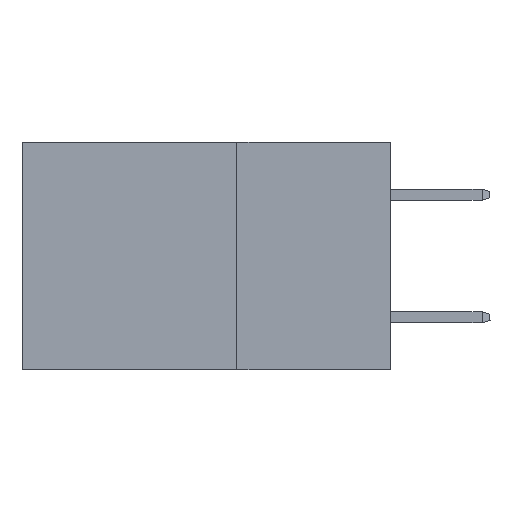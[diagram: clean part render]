
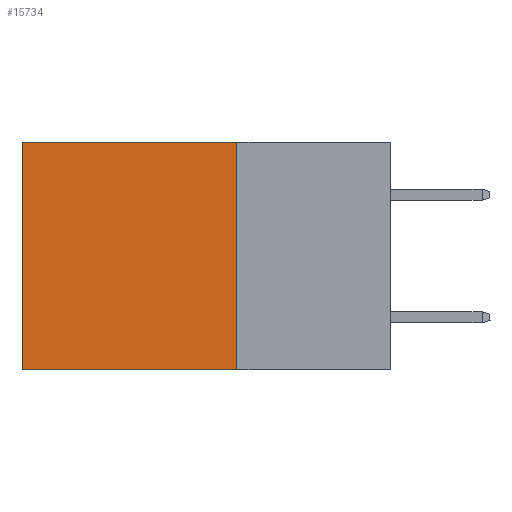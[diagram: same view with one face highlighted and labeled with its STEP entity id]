
A CAD part, left-side view. The second image highlights one B-rep face of the part: STEP entity #15734.
In plain terms, the highlighted planar face has unit normal (-1, 0, 0).
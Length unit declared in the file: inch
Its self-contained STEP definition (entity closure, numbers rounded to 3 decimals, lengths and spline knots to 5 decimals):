
#338 = CARTESIAN_POINT ( 'NONE',  ( 0.2875, 0.6, 0. ) ) ;
#1150 = DIRECTION ( 'NONE',  ( 0., 0., -1. ) ) ;
#3191 = VERTEX_POINT ( 'NONE', #15203 ) ;
#3531 = DIRECTION ( 'NONE',  ( 0., 1., 0. ) ) ;
#3617 = VERTEX_POINT ( 'NONE', #338 ) ;
#3893 = ORIENTED_EDGE ( 'NONE', *, *, #8756, .F. ) ;
#4006 = CARTESIAN_POINT ( 'NONE',  ( 0.2875, 0.6, 0. ) ) ;
#5354 = ORIENTED_EDGE ( 'NONE', *, *, #5396, .F. ) ;
#5396 = EDGE_CURVE ( 'NONE', #3191, #10944, #7378, .T. ) ;
#5787 = PLANE ( 'NONE',  #14468 ) ;
#6396 = DIRECTION ( 'NONE',  ( 0., 0., -1. ) ) ;
#6768 = EDGE_CURVE ( 'NONE', #18883, #3617, #9711, .T. ) ;
#7378 = LINE ( 'NONE', #13441, #19735 ) ;
#7701 = VECTOR ( 'NONE', #6396, 39.37008 ) ;
#7862 = DIRECTION ( 'NONE',  ( 1., 0., 0. ) ) ;
#8206 = EDGE_LOOP ( 'NONE', ( #20328, #5354, #3893, #17914 ) ) ;
#8756 = EDGE_CURVE ( 'NONE', #18883, #3191, #13744, .T. ) ;
#9711 = LINE ( 'NONE', #20864, #19558 ) ;
#10944 = VERTEX_POINT ( 'NONE', #21386 ) ;
#11224 = CARTESIAN_POINT ( 'NONE',  ( 0.2875, 0.25, 0. ) ) ;
#11353 = CARTESIAN_POINT ( 'NONE',  ( 0.2875, 0.25, 0. ) ) ;
#13441 = CARTESIAN_POINT ( 'NONE',  ( 0.2875, 0.25, -0.37 ) ) ;
#13744 = LINE ( 'NONE', #11224, #18980 ) ;
#14468 = AXIS2_PLACEMENT_3D ( 'NONE', #19991, #7862, #20155 ) ;
#15203 = CARTESIAN_POINT ( 'NONE',  ( 0.2875, 0.25, -0.37 ) ) ;
#15734 = ADVANCED_FACE ( 'NONE', ( #17510 ), #5787, .F. ) ;
#17078 = DIRECTION ( 'NONE',  ( 0., 1., 0. ) ) ;
#17510 = FACE_OUTER_BOUND ( 'NONE', #8206, .T. ) ;
#17914 = ORIENTED_EDGE ( 'NONE', *, *, #6768, .T. ) ;
#18242 = EDGE_CURVE ( 'NONE', #3617, #10944, #20066, .T. ) ;
#18883 = VERTEX_POINT ( 'NONE', #11353 ) ;
#18980 = VECTOR ( 'NONE', #1150, 39.37008 ) ;
#19558 = VECTOR ( 'NONE', #3531, 39.37008 ) ;
#19735 = VECTOR ( 'NONE', #17078, 39.37008 ) ;
#19991 = CARTESIAN_POINT ( 'NONE',  ( 0.2875, 0.25, 0. ) ) ;
#20066 = LINE ( 'NONE', #4006, #7701 ) ;
#20155 = DIRECTION ( 'NONE',  ( 0., 0., -1. ) ) ;
#20328 = ORIENTED_EDGE ( 'NONE', *, *, #18242, .T. ) ;
#20864 = CARTESIAN_POINT ( 'NONE',  ( 0.2875, 0.25, 0. ) ) ;
#21386 = CARTESIAN_POINT ( 'NONE',  ( 0.2875, 0.6, -0.37 ) ) ;
